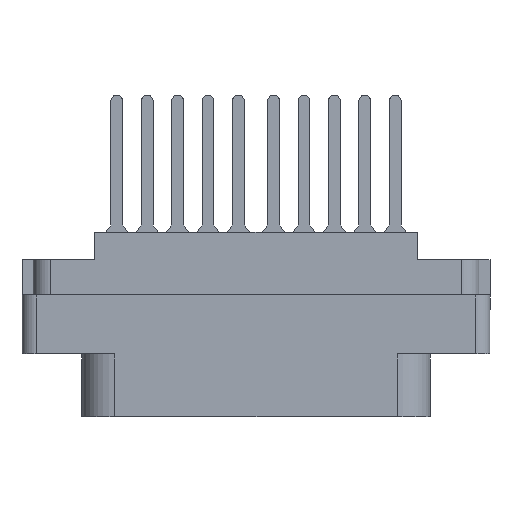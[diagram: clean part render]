
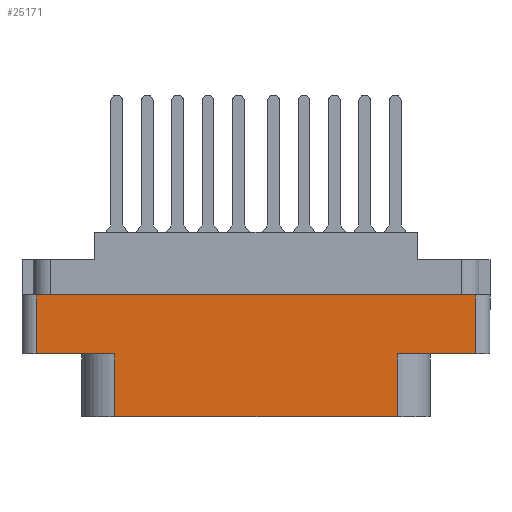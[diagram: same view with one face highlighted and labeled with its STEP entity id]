
A CAD part, front view. The second image highlights one B-rep face of the part: STEP entity #25171.
In plain terms, the highlighted planar face has unit normal (0, -1, 0).
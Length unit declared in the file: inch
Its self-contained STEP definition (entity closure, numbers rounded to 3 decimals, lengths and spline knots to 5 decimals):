
#647 = EDGE_CURVE ( 'NONE', #31680, #11687, #33842, .T. ) ;
#653 = CARTESIAN_POINT ( 'NONE',  ( -0.938, -0.438, -0.789 ) ) ;
#2710 = CARTESIAN_POINT ( 'NONE',  ( 0.604, -0.438, -0.52 ) ) ;
#2833 = DIRECTION ( 'NONE',  ( 0., 0., 1. ) ) ;
#3246 = CARTESIAN_POINT ( 'NONE',  ( 0., -0.438, -0.52 ) ) ;
#3974 = LINE ( 'NONE', #15570, #18102 ) ;
#4533 = LINE ( 'NONE', #14140, #32770 ) ;
#6008 = ORIENTED_EDGE ( 'NONE', *, *, #35888, .T. ) ;
#6560 = CARTESIAN_POINT ( 'NONE',  ( -0.604, -0.438, -0.52 ) ) ;
#6806 = CARTESIAN_POINT ( 'NONE',  ( -0.604, -0.438, -0.789 ) ) ;
#7160 = FACE_OUTER_BOUND ( 'NONE', #24579, .T. ) ;
#7350 = EDGE_CURVE ( 'NONE', #37409, #33902, #24066, .T. ) ;
#7594 = VERTEX_POINT ( 'NONE', #6806 ) ;
#7749 = VECTOR ( 'NONE', #2833, 39.37008 ) ;
#8459 = VERTEX_POINT ( 'NONE', #22553 ) ;
#9003 = ORIENTED_EDGE ( 'NONE', *, *, #30289, .T. ) ;
#9239 = DIRECTION ( 'NONE',  ( 0., -1., 0. ) ) ;
#10850 = LINE ( 'NONE', #653, #28542 ) ;
#10943 = VECTOR ( 'NONE', #11928, 39.37008 ) ;
#11565 = CARTESIAN_POINT ( 'NONE',  ( -0.938, -0.438, -0.268 ) ) ;
#11687 = VERTEX_POINT ( 'NONE', #20114 ) ;
#11928 = DIRECTION ( 'NONE',  ( 1., 0., 0. ) ) ;
#13077 = ORIENTED_EDGE ( 'NONE', *, *, #14622, .T. ) ;
#13212 = AXIS2_PLACEMENT_3D ( 'NONE', #14995, #9239, #20936 ) ;
#14140 = CARTESIAN_POINT ( 'NONE',  ( -0.604, -0.438, -0.789 ) ) ;
#14622 = EDGE_CURVE ( 'NONE', #7594, #31949, #3974, .T. ) ;
#14995 = CARTESIAN_POINT ( 'NONE',  ( -1., -0.438, -0.789 ) ) ;
#15570 = CARTESIAN_POINT ( 'NONE',  ( -1., -0.438, -0.789 ) ) ;
#15952 = DIRECTION ( 'NONE',  ( 1., 0., 0. ) ) ;
#16783 = VECTOR ( 'NONE', #18253, 39.37008 ) ;
#16800 = DIRECTION ( 'NONE',  ( -1., 0., 0. ) ) ;
#17016 = CARTESIAN_POINT ( 'NONE',  ( 0., -0.438, -0.268 ) ) ;
#18102 = VECTOR ( 'NONE', #15952, 39.37008 ) ;
#18211 = DIRECTION ( 'NONE',  ( 0., 0., -1. ) ) ;
#18253 = DIRECTION ( 'NONE',  ( 0., 0., 1. ) ) ;
#19337 = LINE ( 'NONE', #31432, #32105 ) ;
#19442 = ORIENTED_EDGE ( 'NONE', *, *, #7350, .T. ) ;
#20009 = ORIENTED_EDGE ( 'NONE', *, *, #37538, .T. ) ;
#20114 = CARTESIAN_POINT ( 'NONE',  ( 0.938, -0.438, -0.268 ) ) ;
#20936 = DIRECTION ( 'NONE',  ( 0., 0., -1. ) ) ;
#21265 = CARTESIAN_POINT ( 'NONE',  ( 0.604, -0.438, -0.789 ) ) ;
#21706 = ORIENTED_EDGE ( 'NONE', *, *, #31124, .T. ) ;
#22553 = CARTESIAN_POINT ( 'NONE',  ( 0.938, -0.438, -0.52 ) ) ;
#24066 = LINE ( 'NONE', #3246, #10943 ) ;
#24072 = ORIENTED_EDGE ( 'NONE', *, *, #32953, .F. ) ;
#24579 = EDGE_LOOP ( 'NONE', ( #29353, #21706, #19442, #9003, #13077, #6008, #24072, #20009 ) ) ;
#25028 = LINE ( 'NONE', #2710, #7749 ) ;
#25171 = ADVANCED_FACE ( 'NONE', ( #7160 ), #35231, .T. ) ;
#26277 = VERTEX_POINT ( 'NONE', #37666 ) ;
#28109 = LINE ( 'NONE', #33032, #16783 ) ;
#28542 = VECTOR ( 'NONE', #18211, 39.37008 ) ;
#29306 = CARTESIAN_POINT ( 'NONE',  ( -0.938, -0.438, -0.52 ) ) ;
#29353 = ORIENTED_EDGE ( 'NONE', *, *, #647, .F. ) ;
#30289 = EDGE_CURVE ( 'NONE', #33902, #7594, #4533, .T. ) ;
#31124 = EDGE_CURVE ( 'NONE', #31680, #37409, #10850, .T. ) ;
#31432 = CARTESIAN_POINT ( 'NONE',  ( 0., -0.438, -0.52 ) ) ;
#31680 = VERTEX_POINT ( 'NONE', #11565 ) ;
#31949 = VERTEX_POINT ( 'NONE', #21265 ) ;
#32105 = VECTOR ( 'NONE', #16800, 39.37008 ) ;
#32770 = VECTOR ( 'NONE', #34126, 39.37008 ) ;
#32953 = EDGE_CURVE ( 'NONE', #8459, #26277, #19337, .T. ) ;
#33032 = CARTESIAN_POINT ( 'NONE',  ( 0.938, -0.438, -0.789 ) ) ;
#33842 = LINE ( 'NONE', #17016, #36551 ) ;
#33902 = VERTEX_POINT ( 'NONE', #6560 ) ;
#34126 = DIRECTION ( 'NONE',  ( 0., 0., -1. ) ) ;
#35231 = PLANE ( 'NONE',  #13212 ) ;
#35888 = EDGE_CURVE ( 'NONE', #31949, #26277, #25028, .T. ) ;
#36551 = VECTOR ( 'NONE', #37107, 39.37008 ) ;
#37107 = DIRECTION ( 'NONE',  ( 1., 0., 0. ) ) ;
#37409 = VERTEX_POINT ( 'NONE', #29306 ) ;
#37538 = EDGE_CURVE ( 'NONE', #8459, #11687, #28109, .T. ) ;
#37666 = CARTESIAN_POINT ( 'NONE',  ( 0.604, -0.438, -0.52 ) ) ;
